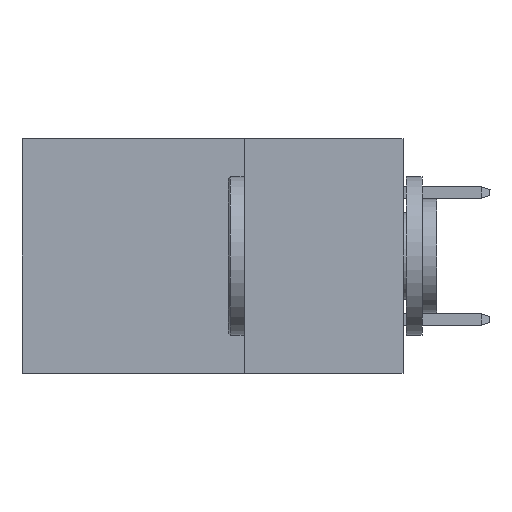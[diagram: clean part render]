
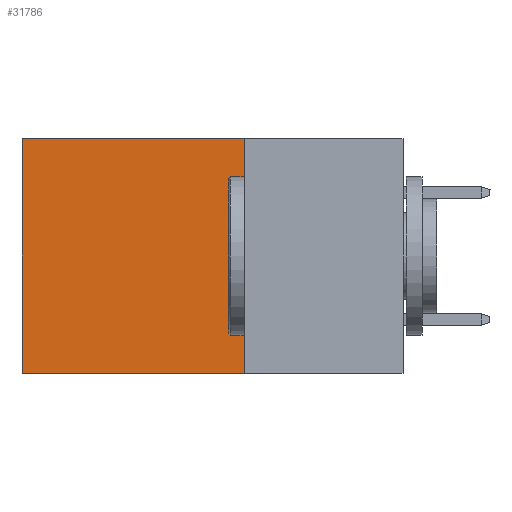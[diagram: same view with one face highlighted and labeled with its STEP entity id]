
A CAD part, left-side view. The second image highlights one B-rep face of the part: STEP entity #31786.
In plain terms, the highlighted planar face has unit normal (-1, 0, 0).
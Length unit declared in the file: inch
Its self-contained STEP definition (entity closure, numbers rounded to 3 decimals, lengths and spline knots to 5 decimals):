
#1837 = CARTESIAN_POINT ( 'NONE',  ( 0.2875, 0.25, 0. ) ) ;
#3070 = DIRECTION ( 'NONE',  ( 0., 0., -1. ) ) ;
#3147 = VERTEX_POINT ( 'NONE', #10865 ) ;
#3393 = ORIENTED_EDGE ( 'NONE', *, *, #4098, .T. ) ;
#4098 = EDGE_CURVE ( 'NONE', #33540, #24884, #23329, .T. ) ;
#10122 = EDGE_LOOP ( 'NONE', ( #27441, #16287, #12821, #3393 ) ) ;
#10865 = CARTESIAN_POINT ( 'NONE',  ( 0.2875, 0.6, -0.37 ) ) ;
#12444 = VECTOR ( 'NONE', #3070, 39.37008 ) ;
#12684 = CARTESIAN_POINT ( 'NONE',  ( 0.2875, 0.6, 0. ) ) ;
#12821 = ORIENTED_EDGE ( 'NONE', *, *, #24374, .F. ) ;
#14321 = CARTESIAN_POINT ( 'NONE',  ( 0.2875, 0.25, 0. ) ) ;
#14856 = AXIS2_PLACEMENT_3D ( 'NONE', #28322, #18720, #24924 ) ;
#16287 = ORIENTED_EDGE ( 'NONE', *, *, #37353, .F. ) ;
#18720 = DIRECTION ( 'NONE',  ( 1., 0., 0. ) ) ;
#18862 = VECTOR ( 'NONE', #19118, 39.37008 ) ;
#19118 = DIRECTION ( 'NONE',  ( 0., 1., 0. ) ) ;
#20427 = VERTEX_POINT ( 'NONE', #25702 ) ;
#22314 = LINE ( 'NONE', #31536, #18862 ) ;
#22616 = CARTESIAN_POINT ( 'NONE',  ( 0.2875, 0.6, 0. ) ) ;
#23329 = LINE ( 'NONE', #14321, #28590 ) ;
#23743 = DIRECTION ( 'NONE',  ( 0., 1., 0. ) ) ;
#24374 = EDGE_CURVE ( 'NONE', #33540, #20427, #29052, .T. ) ;
#24884 = VERTEX_POINT ( 'NONE', #22616 ) ;
#24924 = DIRECTION ( 'NONE',  ( 0., 0., -1. ) ) ;
#25702 = CARTESIAN_POINT ( 'NONE',  ( 0.2875, 0.25, -0.37 ) ) ;
#26248 = DIRECTION ( 'NONE',  ( 0., 0., -1. ) ) ;
#27441 = ORIENTED_EDGE ( 'NONE', *, *, #36412, .T. ) ;
#27528 = FACE_OUTER_BOUND ( 'NONE', #10122, .T. ) ;
#28322 = CARTESIAN_POINT ( 'NONE',  ( 0.2875, 0.25, 0. ) ) ;
#28590 = VECTOR ( 'NONE', #23743, 39.37008 ) ;
#29052 = LINE ( 'NONE', #1837, #33106 ) ;
#31536 = CARTESIAN_POINT ( 'NONE',  ( 0.2875, 0.25, -0.37 ) ) ;
#31786 = ADVANCED_FACE ( 'NONE', ( #27528 ), #37350, .F. ) ;
#33106 = VECTOR ( 'NONE', #26248, 39.37008 ) ;
#33540 = VERTEX_POINT ( 'NONE', #38961 ) ;
#34097 = LINE ( 'NONE', #12684, #12444 ) ;
#36412 = EDGE_CURVE ( 'NONE', #24884, #3147, #34097, .T. ) ;
#37350 = PLANE ( 'NONE',  #14856 ) ;
#37353 = EDGE_CURVE ( 'NONE', #20427, #3147, #22314, .T. ) ;
#38961 = CARTESIAN_POINT ( 'NONE',  ( 0.2875, 0.25, 0. ) ) ;
